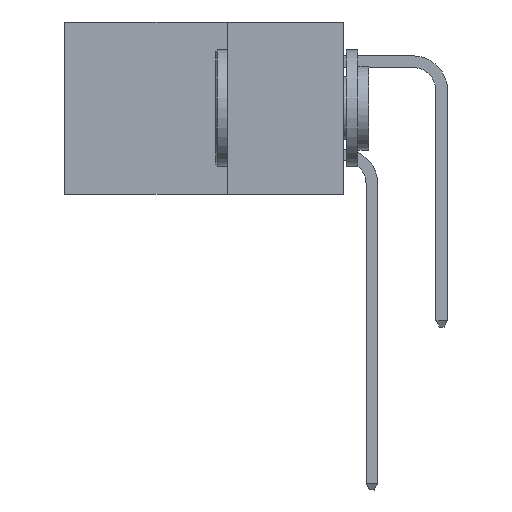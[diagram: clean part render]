
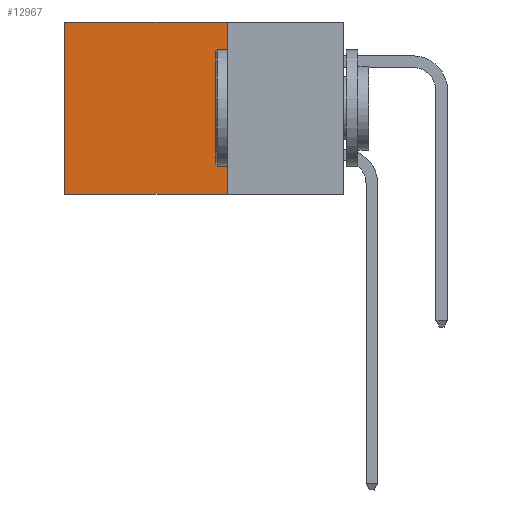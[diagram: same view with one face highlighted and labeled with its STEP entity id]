
A CAD part, left-side view. The second image highlights one B-rep face of the part: STEP entity #12967.
In plain terms, the highlighted planar face has unit normal (-1, 0, 0).
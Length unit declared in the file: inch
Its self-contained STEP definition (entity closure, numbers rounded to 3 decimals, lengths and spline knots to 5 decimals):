
#193 = CARTESIAN_POINT ( 'NONE',  ( 0.2615, 0.25, -0.37 ) ) ;
#212 = DIRECTION ( 'NONE',  ( 0., 0., -1. ) ) ;
#735 = VECTOR ( 'NONE', #2245, 39.37008 ) ;
#836 = CARTESIAN_POINT ( 'NONE',  ( 0.2615, 0.25, 0. ) ) ;
#1450 = EDGE_CURVE ( 'NONE', #18070, #11572, #7813, .T. ) ;
#1691 = CARTESIAN_POINT ( 'NONE',  ( 0.2615, 0.25, -0.37 ) ) ;
#1911 = CARTESIAN_POINT ( 'NONE',  ( 0.2615, 0.6, -0.37 ) ) ;
#2142 = LINE ( 'NONE', #17835, #8979 ) ;
#2245 = DIRECTION ( 'NONE',  ( 0., 1., 0. ) ) ;
#2775 = VERTEX_POINT ( 'NONE', #6092 ) ;
#3486 = DIRECTION ( 'NONE',  ( 0., 0., -1. ) ) ;
#6092 = CARTESIAN_POINT ( 'NONE',  ( 0.2615, 0.25, -0.37 ) ) ;
#6595 = ORIENTED_EDGE ( 'NONE', *, *, #1450, .T. ) ;
#7337 = ORIENTED_EDGE ( 'NONE', *, *, #18603, .T. ) ;
#7813 = LINE ( 'NONE', #11296, #22988 ) ;
#8918 = EDGE_LOOP ( 'NONE', ( #6595, #24453, #15388, #7337 ) ) ;
#8979 = VECTOR ( 'NONE', #212, 39.37008 ) ;
#9391 = CARTESIAN_POINT ( 'NONE',  ( 0.2615, 0.25, 0. ) ) ;
#9572 = EDGE_CURVE ( 'NONE', #15294, #2775, #2142, .T. ) ;
#9614 = DIRECTION ( 'NONE',  ( 1., 0., 0. ) ) ;
#10294 = LINE ( 'NONE', #193, #735 ) ;
#11296 = CARTESIAN_POINT ( 'NONE',  ( 0.2615, 0.6, -0.37 ) ) ;
#11572 = VERTEX_POINT ( 'NONE', #1911 ) ;
#12967 = ADVANCED_FACE ( 'NONE', ( #17378 ), #17501, .F. ) ;
#15294 = VERTEX_POINT ( 'NONE', #836 ) ;
#15388 = ORIENTED_EDGE ( 'NONE', *, *, #9572, .F. ) ;
#15565 = EDGE_CURVE ( 'NONE', #2775, #11572, #10294, .T. ) ;
#17378 = FACE_OUTER_BOUND ( 'NONE', #8918, .T. ) ;
#17411 = DIRECTION ( 'NONE',  ( 0., 1., 0. ) ) ;
#17501 = PLANE ( 'NONE',  #24054 ) ;
#17835 = CARTESIAN_POINT ( 'NONE',  ( 0.2615, 0.25, -0.37 ) ) ;
#18070 = VERTEX_POINT ( 'NONE', #24799 ) ;
#18603 = EDGE_CURVE ( 'NONE', #15294, #18070, #21252, .T. ) ;
#21252 = LINE ( 'NONE', #9391, #23836 ) ;
#22988 = VECTOR ( 'NONE', #23278, 39.37008 ) ;
#23278 = DIRECTION ( 'NONE',  ( 0., 0., -1. ) ) ;
#23836 = VECTOR ( 'NONE', #17411, 39.37008 ) ;
#24054 = AXIS2_PLACEMENT_3D ( 'NONE', #1691, #9614, #3486 ) ;
#24453 = ORIENTED_EDGE ( 'NONE', *, *, #15565, .F. ) ;
#24799 = CARTESIAN_POINT ( 'NONE',  ( 0.2615, 0.6, 0. ) ) ;
